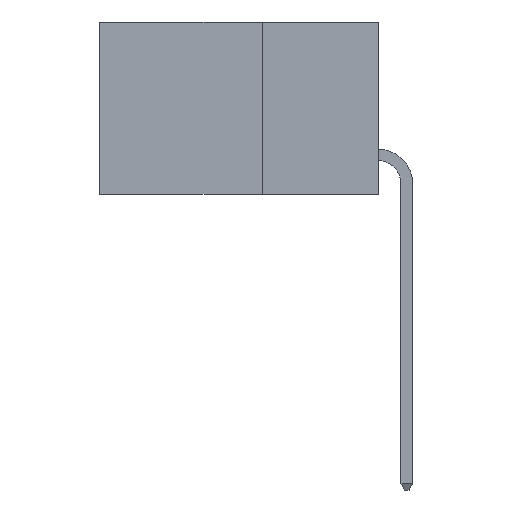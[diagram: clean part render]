
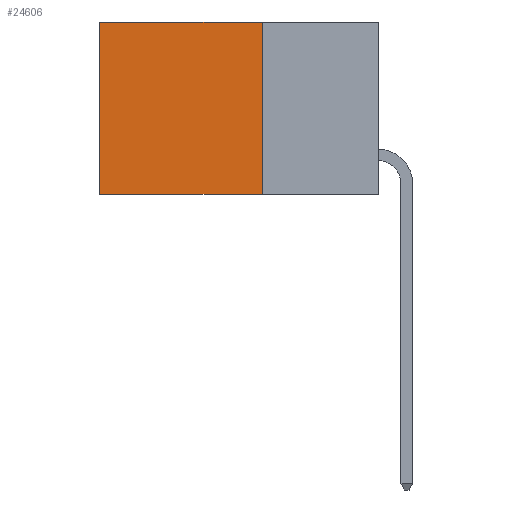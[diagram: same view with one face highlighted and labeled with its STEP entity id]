
A CAD part, left-side view. The second image highlights one B-rep face of the part: STEP entity #24606.
In plain terms, the highlighted planar face has unit normal (-1, 0, 0).
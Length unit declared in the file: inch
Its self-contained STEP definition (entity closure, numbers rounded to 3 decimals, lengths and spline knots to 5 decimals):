
#396 = DIRECTION ( 'NONE',  ( 1., 0., 0. ) ) ;
#486 = EDGE_CURVE ( 'NONE', #5165, #11261, #8050, .T. ) ;
#2360 = VECTOR ( 'NONE', #14694, 39.37008 ) ;
#3015 = LINE ( 'NONE', #14877, #2360 ) ;
#4920 = CARTESIAN_POINT ( 'NONE',  ( 0.2615, 0.25, 0. ) ) ;
#5165 = VERTEX_POINT ( 'NONE', #4920 ) ;
#6267 = VERTEX_POINT ( 'NONE', #21807 ) ;
#6692 = VECTOR ( 'NONE', #13557, 39.37008 ) ;
#8050 = LINE ( 'NONE', #12958, #18689 ) ;
#8212 = EDGE_CURVE ( 'NONE', #5165, #24006, #3015, .T. ) ;
#8310 = EDGE_LOOP ( 'NONE', ( #10826, #12780, #19792, #25561 ) ) ;
#10350 = AXIS2_PLACEMENT_3D ( 'NONE', #24501, #396, #14558 ) ;
#10559 = PLANE ( 'NONE',  #10350 ) ;
#10817 = EDGE_CURVE ( 'NONE', #24006, #6267, #23278, .T. ) ;
#10826 = ORIENTED_EDGE ( 'NONE', *, *, #12192, .T. ) ;
#11261 = VERTEX_POINT ( 'NONE', #16805 ) ;
#12192 = EDGE_CURVE ( 'NONE', #11261, #6267, #25317, .T. ) ;
#12502 = DIRECTION ( 'NONE',  ( 0., 1., 0. ) ) ;
#12780 = ORIENTED_EDGE ( 'NONE', *, *, #10817, .F. ) ;
#12958 = CARTESIAN_POINT ( 'NONE',  ( 0.2615, 0.25, 0. ) ) ;
#13557 = DIRECTION ( 'NONE',  ( 0., 1., 0. ) ) ;
#14558 = DIRECTION ( 'NONE',  ( 0., 0., -1. ) ) ;
#14694 = DIRECTION ( 'NONE',  ( 0., 0., -1. ) ) ;
#14740 = VECTOR ( 'NONE', #19456, 39.37008 ) ;
#14877 = CARTESIAN_POINT ( 'NONE',  ( 0.2615, 0.25, -0.37 ) ) ;
#16805 = CARTESIAN_POINT ( 'NONE',  ( 0.2615, 0.6, 0. ) ) ;
#18679 = FACE_OUTER_BOUND ( 'NONE', #8310, .T. ) ;
#18689 = VECTOR ( 'NONE', #12502, 39.37008 ) ;
#19456 = DIRECTION ( 'NONE',  ( 0., 0., -1. ) ) ;
#19630 = CARTESIAN_POINT ( 'NONE',  ( 0.2615, 0.25, -0.37 ) ) ;
#19792 = ORIENTED_EDGE ( 'NONE', *, *, #8212, .F. ) ;
#21553 = CARTESIAN_POINT ( 'NONE',  ( 0.2615, 0.6, -0.37 ) ) ;
#21807 = CARTESIAN_POINT ( 'NONE',  ( 0.2615, 0.6, -0.37 ) ) ;
#22746 = CARTESIAN_POINT ( 'NONE',  ( 0.2615, 0.25, -0.37 ) ) ;
#23278 = LINE ( 'NONE', #19630, #6692 ) ;
#24006 = VERTEX_POINT ( 'NONE', #22746 ) ;
#24501 = CARTESIAN_POINT ( 'NONE',  ( 0.2615, 0.25, -0.37 ) ) ;
#24606 = ADVANCED_FACE ( 'NONE', ( #18679 ), #10559, .F. ) ;
#25317 = LINE ( 'NONE', #21553, #14740 ) ;
#25561 = ORIENTED_EDGE ( 'NONE', *, *, #486, .T. ) ;
